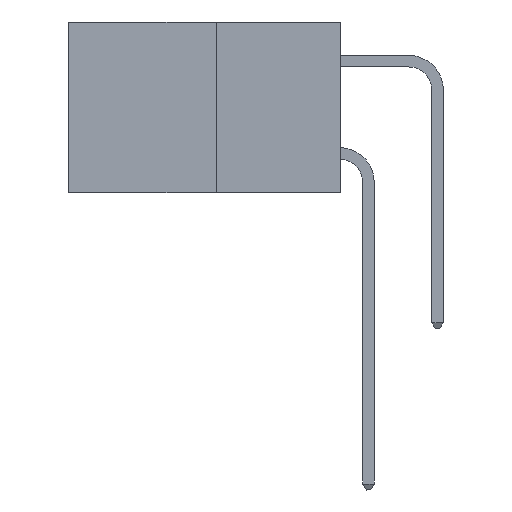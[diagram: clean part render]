
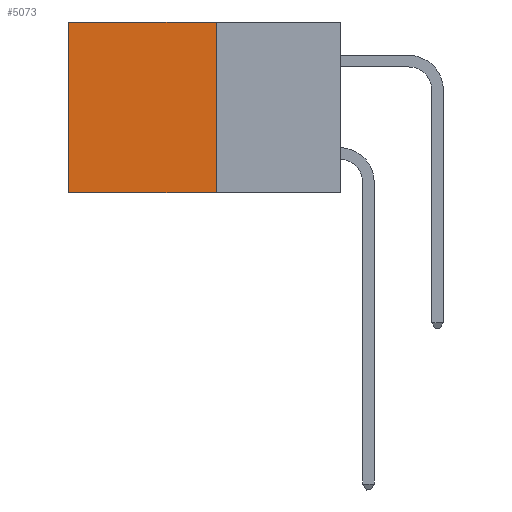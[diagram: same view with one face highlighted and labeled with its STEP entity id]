
A CAD part, left-side view. The second image highlights one B-rep face of the part: STEP entity #5073.
In plain terms, the highlighted planar face has unit normal (-1, 0, 0).
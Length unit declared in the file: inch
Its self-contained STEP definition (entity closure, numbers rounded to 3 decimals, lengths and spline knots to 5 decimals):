
#822 = EDGE_CURVE ( 'NONE', #8411, #10400, #8138, .T. ) ;
#1644 = EDGE_CURVE ( 'NONE', #5025, #8411, #20689, .T. ) ;
#2004 = ORIENTED_EDGE ( 'NONE', *, *, #15088, .T. ) ;
#2133 = ORIENTED_EDGE ( 'NONE', *, *, #1644, .F. ) ;
#3592 = ORIENTED_EDGE ( 'NONE', *, *, #822, .F. ) ;
#3676 = VECTOR ( 'NONE', #17489, 39.37008 ) ;
#3790 = ORIENTED_EDGE ( 'NONE', *, *, #7710, .T. ) ;
#4803 = CARTESIAN_POINT ( 'NONE',  ( 0.277, 0.59, 0. ) ) ;
#5025 = VERTEX_POINT ( 'NONE', #21414 ) ;
#5073 = ADVANCED_FACE ( 'NONE', ( #12553 ), #13830, .F. ) ;
#6385 = DIRECTION ( 'NONE',  ( 0., 1., 0. ) ) ;
#6541 = CARTESIAN_POINT ( 'NONE',  ( 0.277, 0.27, 0. ) ) ;
#7594 = VECTOR ( 'NONE', #10195, 39.37008 ) ;
#7598 = AXIS2_PLACEMENT_3D ( 'NONE', #11057, #14815, #14783 ) ;
#7710 = EDGE_CURVE ( 'NONE', #9576, #10400, #12170, .T. ) ;
#8138 = LINE ( 'NONE', #14245, #20734 ) ;
#8411 = VERTEX_POINT ( 'NONE', #9614 ) ;
#9576 = VERTEX_POINT ( 'NONE', #4803 ) ;
#9614 = CARTESIAN_POINT ( 'NONE',  ( 0.277, 0.27, -0.37 ) ) ;
#10048 = LINE ( 'NONE', #6541, #18208 ) ;
#10126 = CARTESIAN_POINT ( 'NONE',  ( 0.277, 0.27, -0.37 ) ) ;
#10195 = DIRECTION ( 'NONE',  ( 0., 0., -1. ) ) ;
#10400 = VERTEX_POINT ( 'NONE', #11989 ) ;
#11057 = CARTESIAN_POINT ( 'NONE',  ( 0.277, 0.27, -0.37 ) ) ;
#11989 = CARTESIAN_POINT ( 'NONE',  ( 0.277, 0.59, -0.37 ) ) ;
#12170 = LINE ( 'NONE', #17549, #3676 ) ;
#12553 = FACE_OUTER_BOUND ( 'NONE', #15449, .T. ) ;
#13619 = DIRECTION ( 'NONE',  ( 0., 1., 0. ) ) ;
#13830 = PLANE ( 'NONE',  #7598 ) ;
#14245 = CARTESIAN_POINT ( 'NONE',  ( 0.277, 0.27, -0.37 ) ) ;
#14783 = DIRECTION ( 'NONE',  ( 0., 0., -1. ) ) ;
#14815 = DIRECTION ( 'NONE',  ( 1., 0., 0. ) ) ;
#15088 = EDGE_CURVE ( 'NONE', #5025, #9576, #10048, .T. ) ;
#15449 = EDGE_LOOP ( 'NONE', ( #3790, #3592, #2133, #2004 ) ) ;
#17489 = DIRECTION ( 'NONE',  ( 0., 0., -1. ) ) ;
#17549 = CARTESIAN_POINT ( 'NONE',  ( 0.277, 0.59, -0.37 ) ) ;
#18208 = VECTOR ( 'NONE', #6385, 39.37008 ) ;
#20689 = LINE ( 'NONE', #10126, #7594 ) ;
#20734 = VECTOR ( 'NONE', #13619, 39.37008 ) ;
#21414 = CARTESIAN_POINT ( 'NONE',  ( 0.277, 0.27, 0. ) ) ;
